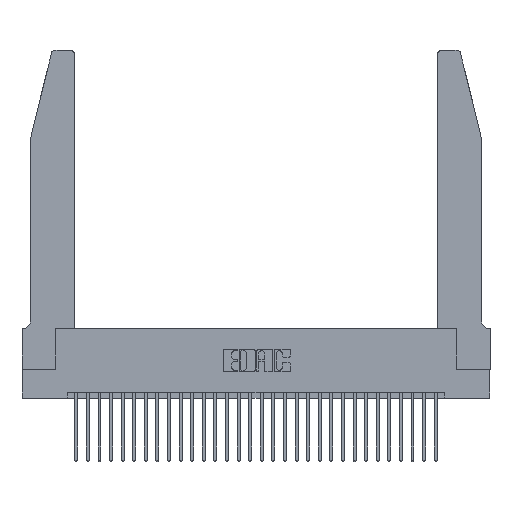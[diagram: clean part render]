
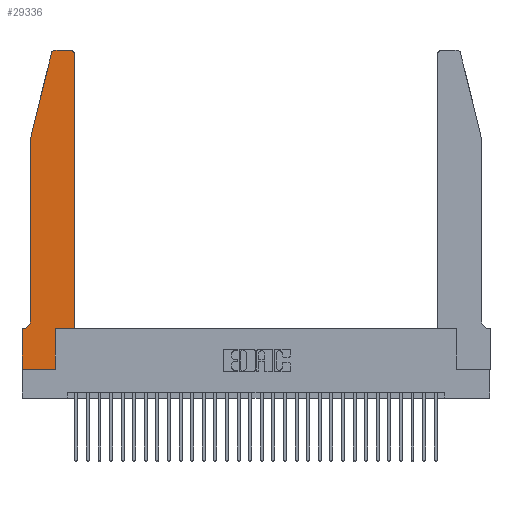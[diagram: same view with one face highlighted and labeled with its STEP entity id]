
A CAD part, top view. The second image highlights one B-rep face of the part: STEP entity #29336.
In plain terms, the highlighted planar face has unit normal (0, 0, 1).
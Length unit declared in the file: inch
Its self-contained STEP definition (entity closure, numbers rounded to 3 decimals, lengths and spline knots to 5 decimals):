
#47 = CARTESIAN_POINT ( 'NONE',  ( 0.0755, 2., 0.37 ) ) ;
#93 = CARTESIAN_POINT ( 'NONE',  ( 0.2605, 2.75, 0.37 ) ) ;
#183 = CARTESIAN_POINT ( 'NONE',  ( 0.2865, 0., 0.37 ) ) ;
#269 = DIRECTION ( 'NONE',  ( 1., 0., 0. ) ) ;
#373 = DIRECTION ( 'NONE',  ( 0., 0., 1. ) ) ;
#736 = DIRECTION ( 'NONE',  ( 0., -1., 0. ) ) ;
#1268 = VERTEX_POINT ( 'NONE', #25230 ) ;
#1434 = DIRECTION ( 'NONE',  ( 0., 1., 0. ) ) ;
#1773 = ORIENTED_EDGE ( 'NONE', *, *, #14097, .T. ) ;
#1981 = AXIS2_PLACEMENT_3D ( 'NONE', #16099, #20626, #8735 ) ;
#2015 = CARTESIAN_POINT ( 'NONE',  ( 0.4205, 2.72, 0.37 ) ) ;
#2398 = CARTESIAN_POINT ( 'NONE',  ( 0.0055, 0.35, 0.37 ) ) ;
#2914 = CARTESIAN_POINT ( 'NONE',  ( 0.4505, 0.35, 0.37 ) ) ;
#3215 = VERTEX_POINT ( 'NONE', #8779 ) ;
#3839 = CARTESIAN_POINT ( 'NONE',  ( 0.25487, 2.72718, 0.37 ) ) ;
#4045 = PLANE ( 'NONE',  #1981 ) ;
#4406 = DIRECTION ( 'NONE',  ( 0., 0., 1. ) ) ;
#4560 = AXIS2_PLACEMENT_3D ( 'NONE', #17058, #373, #269 ) ;
#4774 = LINE ( 'NONE', #30646, #9711 ) ;
#4849 = ORIENTED_EDGE ( 'NONE', *, *, #8075, .T. ) ;
#5611 = DIRECTION ( 'NONE',  ( 0., 1., 0. ) ) ;
#6864 = DIRECTION ( 'NONE',  ( 1., 0., 0. ) ) ;
#6974 = CARTESIAN_POINT ( 'NONE',  ( 0.0755, 0.42, 0.37 ) ) ;
#7037 = CARTESIAN_POINT ( 'NONE',  ( 0.2865, 0.35, 0.37 ) ) ;
#7762 = AXIS2_PLACEMENT_3D ( 'NONE', #2015, #4406, #6864 ) ;
#8075 = EDGE_CURVE ( 'NONE', #15513, #1268, #14323, .T. ) ;
#8184 = EDGE_CURVE ( 'NONE', #30277, #15513, #19969, .T. ) ;
#8248 = VERTEX_POINT ( 'NONE', #24322 ) ;
#8514 = CARTESIAN_POINT ( 'NONE',  ( 0.4505, 0.35, 0.37 ) ) ;
#8735 = DIRECTION ( 'NONE',  ( 1., 0., 0. ) ) ;
#8779 = CARTESIAN_POINT ( 'NONE',  ( 0.4205, 2.75, 0.37 ) ) ;
#9422 = EDGE_CURVE ( 'NONE', #22277, #8248, #16114, .T. ) ;
#9711 = VECTOR ( 'NONE', #23688, 39.37008 ) ;
#10776 = DIRECTION ( 'NONE',  ( 1., 0., 0. ) ) ;
#10803 = AXIS2_PLACEMENT_3D ( 'NONE', #11442, #16176, #20910 ) ;
#10982 = EDGE_CURVE ( 'NONE', #15373, #14927, #11140, .T. ) ;
#11140 = LINE ( 'NONE', #8514, #29590 ) ;
#11386 = EDGE_LOOP ( 'NONE', ( #18639, #29697, #4849, #19207, #22674, #24801, #28846, #27039, #23405, #1773, #28559, #25369 ) ) ;
#11442 = CARTESIAN_POINT ( 'NONE',  ( 0.0055, 0.42, 0.37 ) ) ;
#12512 = VERTEX_POINT ( 'NONE', #18599 ) ;
#13614 = EDGE_CURVE ( 'NONE', #1268, #17775, #27933, .T. ) ;
#13806 = CARTESIAN_POINT ( 'NONE',  ( 0.4505, 2.72, 0.37 ) ) ;
#14097 = EDGE_CURVE ( 'NONE', #27017, #15373, #20346, .T. ) ;
#14323 = LINE ( 'NONE', #47, #18483 ) ;
#14496 = EDGE_CURVE ( 'NONE', #12512, #24793, #23021, .T. ) ;
#14627 = LINE ( 'NONE', #20083, #26678 ) ;
#14693 = DIRECTION ( 'NONE',  ( -0.239, -0.971, 0. ) ) ;
#14721 = CARTESIAN_POINT ( 'NONE',  ( 0., 0., 0.37 ) ) ;
#14927 = VERTEX_POINT ( 'NONE', #13806 ) ;
#15373 = VERTEX_POINT ( 'NONE', #2914 ) ;
#15513 = VERTEX_POINT ( 'NONE', #3839 ) ;
#15922 = EDGE_CURVE ( 'NONE', #14927, #3215, #17283, .T. ) ;
#16099 = CARTESIAN_POINT ( 'NONE',  ( 0., 0.35, 0.37 ) ) ;
#16114 = LINE ( 'NONE', #24577, #17263 ) ;
#16176 = DIRECTION ( 'NONE',  ( 0., 0., -1. ) ) ;
#16254 = VECTOR ( 'NONE', #736, 39.37008 ) ;
#16788 = DIRECTION ( 'NONE',  ( 1., 0., 0. ) ) ;
#16869 = DIRECTION ( 'NONE',  ( -1., 0., 0. ) ) ;
#16985 = VECTOR ( 'NONE', #10776, 39.37008 ) ;
#17058 = CARTESIAN_POINT ( 'NONE',  ( 0.284, 2.72, 0.37 ) ) ;
#17068 = LINE ( 'NONE', #93, #28760 ) ;
#17263 = VECTOR ( 'NONE', #29413, 39.37008 ) ;
#17283 = CIRCLE ( 'NONE', #7762, 0.03 ) ;
#17775 = VERTEX_POINT ( 'NONE', #6974 ) ;
#18140 = VECTOR ( 'NONE', #16788, 39.37008 ) ;
#18483 = VECTOR ( 'NONE', #14693, 39.37008 ) ;
#18523 = FACE_OUTER_BOUND ( 'NONE', #11386, .T. ) ;
#18599 = CARTESIAN_POINT ( 'NONE',  ( 0., 0., 0.37 ) ) ;
#18639 = ORIENTED_EDGE ( 'NONE', *, *, #28388, .T. ) ;
#19207 = ORIENTED_EDGE ( 'NONE', *, *, #13614, .T. ) ;
#19333 = CARTESIAN_POINT ( 'NONE',  ( 0.284, 2.75, 0.37 ) ) ;
#19969 = CIRCLE ( 'NONE', #4560, 0.03 ) ;
#20083 = CARTESIAN_POINT ( 'NONE',  ( 0.2865, 0.35, 0.37 ) ) ;
#20346 = LINE ( 'NONE', #22772, #16985 ) ;
#20626 = DIRECTION ( 'NONE',  ( 0., 0., 1. ) ) ;
#20910 = DIRECTION ( 'NONE',  ( -1., 0., 0. ) ) ;
#22277 = VERTEX_POINT ( 'NONE', #2398 ) ;
#22674 = ORIENTED_EDGE ( 'NONE', *, *, #25227, .T. ) ;
#22772 = CARTESIAN_POINT ( 'NONE',  ( 0.4505, 0.35, 0.37 ) ) ;
#23021 = LINE ( 'NONE', #14721, #18140 ) ;
#23405 = ORIENTED_EDGE ( 'NONE', *, *, #24977, .T. ) ;
#23688 = DIRECTION ( 'NONE',  ( 0., -1., 0. ) ) ;
#24322 = CARTESIAN_POINT ( 'NONE',  ( 0., 0.35, 0.37 ) ) ;
#24577 = CARTESIAN_POINT ( 'NONE',  ( 0.0755, 0.35, 0.37 ) ) ;
#24793 = VERTEX_POINT ( 'NONE', #183 ) ;
#24795 = EDGE_CURVE ( 'NONE', #8248, #12512, #4774, .T. ) ;
#24801 = ORIENTED_EDGE ( 'NONE', *, *, #9422, .T. ) ;
#24977 = EDGE_CURVE ( 'NONE', #24793, #27017, #14627, .T. ) ;
#25227 = EDGE_CURVE ( 'NONE', #17775, #22277, #29316, .T. ) ;
#25230 = CARTESIAN_POINT ( 'NONE',  ( 0.0755, 2., 0.37 ) ) ;
#25369 = ORIENTED_EDGE ( 'NONE', *, *, #15922, .T. ) ;
#26678 = VECTOR ( 'NONE', #5611, 39.37008 ) ;
#27017 = VERTEX_POINT ( 'NONE', #7037 ) ;
#27039 = ORIENTED_EDGE ( 'NONE', *, *, #14496, .T. ) ;
#27933 = LINE ( 'NONE', #29628, #16254 ) ;
#28388 = EDGE_CURVE ( 'NONE', #3215, #30277, #17068, .T. ) ;
#28559 = ORIENTED_EDGE ( 'NONE', *, *, #10982, .T. ) ;
#28760 = VECTOR ( 'NONE', #16869, 39.37008 ) ;
#28846 = ORIENTED_EDGE ( 'NONE', *, *, #24795, .T. ) ;
#29316 = CIRCLE ( 'NONE', #10803, 0.07 ) ;
#29336 = ADVANCED_FACE ( 'NONE', ( #18523 ), #4045, .T. ) ;
#29413 = DIRECTION ( 'NONE',  ( -1., 0., 0. ) ) ;
#29590 = VECTOR ( 'NONE', #1434, 39.37008 ) ;
#29628 = CARTESIAN_POINT ( 'NONE',  ( 0.0755, 2., 0.37 ) ) ;
#29697 = ORIENTED_EDGE ( 'NONE', *, *, #8184, .T. ) ;
#30277 = VERTEX_POINT ( 'NONE', #19333 ) ;
#30646 = CARTESIAN_POINT ( 'NONE',  ( 0., 0., 0.37 ) ) ;
